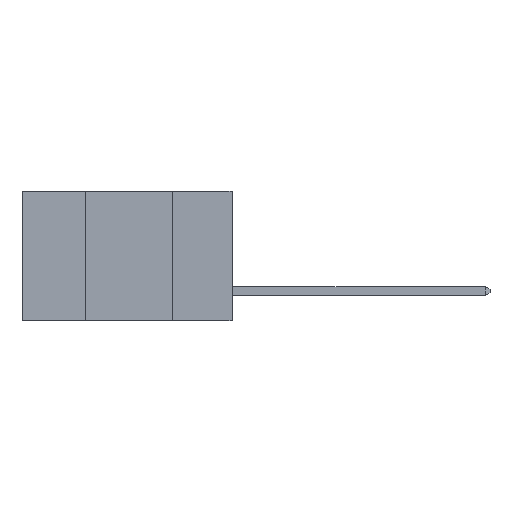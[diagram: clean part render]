
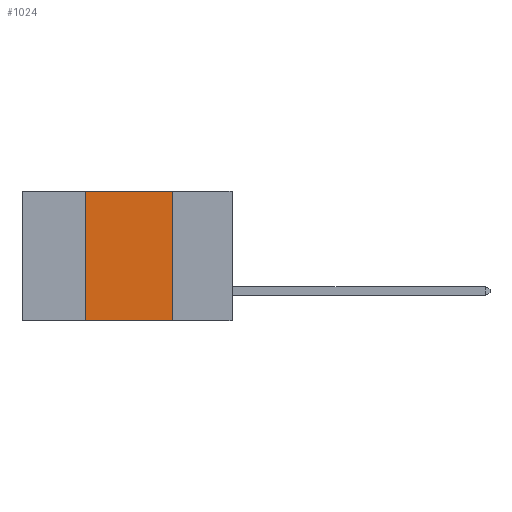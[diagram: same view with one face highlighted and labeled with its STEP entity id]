
A CAD part, left-side view. The second image highlights one B-rep face of the part: STEP entity #1024.
In plain terms, the highlighted planar face has unit normal (-1, 0, 0).
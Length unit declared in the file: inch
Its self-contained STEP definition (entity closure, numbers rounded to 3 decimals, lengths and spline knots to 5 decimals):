
#82 = CARTESIAN_POINT ( 'NONE',  ( 0., 0.6, 0. ) ) ;
#376 = PLANE ( 'NONE',  #3004 ) ;
#648 = EDGE_CURVE ( 'NONE', #2690, #2799, #11859, .T. ) ;
#679 = CARTESIAN_POINT ( 'NONE',  ( 0., 0.6, 0. ) ) ;
#826 = FACE_OUTER_BOUND ( 'NONE', #1413, .T. ) ;
#1024 = ADVANCED_FACE ( 'NONE', ( #826 ), #376, .F. ) ;
#1311 = CARTESIAN_POINT ( 'NONE',  ( 0., 0.42, -0.37 ) ) ;
#1413 = EDGE_LOOP ( 'NONE', ( #11761, #11777, #11846, #11905 ) ) ;
#1792 = DIRECTION ( 'NONE',  ( 0., -1., 0. ) ) ;
#1903 = VERTEX_POINT ( 'NONE', #11069 ) ;
#2400 = DIRECTION ( 'NONE',  ( 1., 0., 0. ) ) ;
#2495 = VECTOR ( 'NONE', #5653, 39.37008 ) ;
#2534 = VECTOR ( 'NONE', #6496, 39.37008 ) ;
#2690 = VERTEX_POINT ( 'NONE', #1311 ) ;
#2799 = VERTEX_POINT ( 'NONE', #10518 ) ;
#2853 = DIRECTION ( 'NONE',  ( 0., 0., 1. ) ) ;
#2882 = CARTESIAN_POINT ( 'NONE',  ( 0., 0.42, 0. ) ) ;
#3004 = AXIS2_PLACEMENT_3D ( 'NONE', #82, #2400, #3401 ) ;
#3401 = DIRECTION ( 'NONE',  ( 0., 0., -1. ) ) ;
#4629 = VERTEX_POINT ( 'NONE', #8086 ) ;
#4924 = LINE ( 'NONE', #679, #10135 ) ;
#5053 = EDGE_CURVE ( 'NONE', #1903, #2799, #10106, .T. ) ;
#5505 = EDGE_CURVE ( 'NONE', #2690, #4629, #9780, .T. ) ;
#5653 = DIRECTION ( 'NONE',  ( 0., 0., -1. ) ) ;
#5677 = CARTESIAN_POINT ( 'NONE',  ( 0., 0.17, 0. ) ) ;
#6496 = DIRECTION ( 'NONE',  ( 0., -1., 0. ) ) ;
#8086 = CARTESIAN_POINT ( 'NONE',  ( 0., 0.42, 0. ) ) ;
#9780 = LINE ( 'NONE', #2882, #12119 ) ;
#10106 = LINE ( 'NONE', #5677, #2495 ) ;
#10135 = VECTOR ( 'NONE', #1792, 39.37008 ) ;
#10518 = CARTESIAN_POINT ( 'NONE',  ( 0., 0.17, -0.37 ) ) ;
#11038 = CARTESIAN_POINT ( 'NONE',  ( 0., 0.6, -0.37 ) ) ;
#11069 = CARTESIAN_POINT ( 'NONE',  ( 0., 0.17, 0. ) ) ;
#11761 = ORIENTED_EDGE ( 'NONE', *, *, #5053, .F. ) ;
#11777 = ORIENTED_EDGE ( 'NONE', *, *, #12004, .F. ) ;
#11846 = ORIENTED_EDGE ( 'NONE', *, *, #5505, .F. ) ;
#11859 = LINE ( 'NONE', #11038, #2534 ) ;
#11905 = ORIENTED_EDGE ( 'NONE', *, *, #648, .T. ) ;
#12004 = EDGE_CURVE ( 'NONE', #4629, #1903, #4924, .T. ) ;
#12119 = VECTOR ( 'NONE', #2853, 39.37008 ) ;
